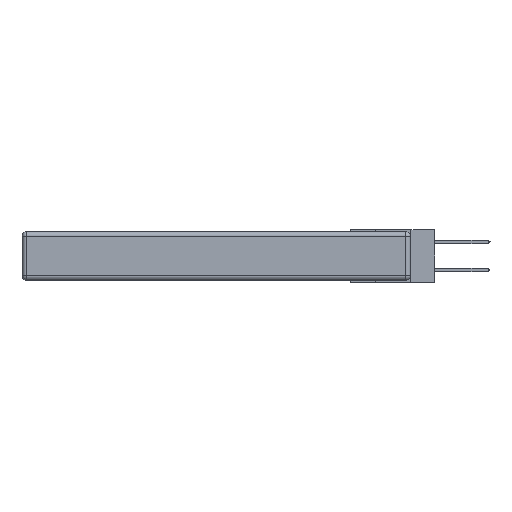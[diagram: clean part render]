
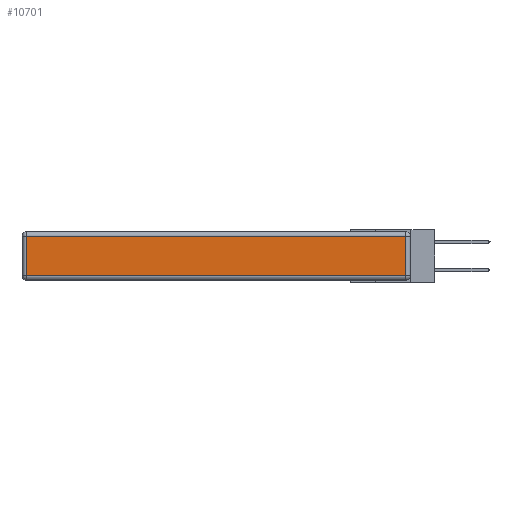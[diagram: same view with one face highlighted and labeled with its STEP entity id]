
A CAD part, left-side view. The second image highlights one B-rep face of the part: STEP entity #10701.
In plain terms, the highlighted planar face has unit normal (-1, 0, 0).
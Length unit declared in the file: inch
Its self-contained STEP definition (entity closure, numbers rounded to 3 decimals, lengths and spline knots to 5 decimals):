
#21 = VECTOR ( 'NONE', #9595, 39.37008 ) ;
#179 = EDGE_CURVE ( 'NONE', #8770, #10755, #1610, .T. ) ;
#392 = VECTOR ( 'NONE', #9634, 39.37008 ) ;
#1179 = EDGE_LOOP ( 'NONE', ( #4653, #8578, #7617, #9391 ) ) ;
#1444 = DIRECTION ( 'NONE',  ( 0., 0., 1. ) ) ;
#1610 = LINE ( 'NONE', #1983, #392 ) ;
#1983 = CARTESIAN_POINT ( 'NONE',  ( 0., 2.72, -0.343 ) ) ;
#4003 = LINE ( 'NONE', #9687, #13252 ) ;
#4013 = CARTESIAN_POINT ( 'NONE',  ( 0., 0.03, -0.313 ) ) ;
#4406 = DIRECTION ( 'NONE',  ( 0., 1., 0. ) ) ;
#4653 = ORIENTED_EDGE ( 'NONE', *, *, #6406, .T. ) ;
#4822 = AXIS2_PLACEMENT_3D ( 'NONE', #11299, #12381, #1444 ) ;
#5662 = PLANE ( 'NONE',  #4822 ) ;
#6313 = LINE ( 'NONE', #11982, #13309 ) ;
#6406 = EDGE_CURVE ( 'NONE', #10755, #13877, #7732, .T. ) ;
#6675 = CARTESIAN_POINT ( 'NONE',  ( 0., 0.03, -0.03 ) ) ;
#7079 = CARTESIAN_POINT ( 'NONE',  ( 0., 2.72, -0.313 ) ) ;
#7617 = ORIENTED_EDGE ( 'NONE', *, *, #10824, .T. ) ;
#7732 = LINE ( 'NONE', #11595, #21 ) ;
#8578 = ORIENTED_EDGE ( 'NONE', *, *, #14036, .T. ) ;
#8770 = VERTEX_POINT ( 'NONE', #10981 ) ;
#9340 = FACE_OUTER_BOUND ( 'NONE', #1179, .T. ) ;
#9391 = ORIENTED_EDGE ( 'NONE', *, *, #179, .T. ) ;
#9595 = DIRECTION ( 'NONE',  ( 0., -1., 0. ) ) ;
#9634 = DIRECTION ( 'NONE',  ( 0., 0., -1. ) ) ;
#9687 = CARTESIAN_POINT ( 'NONE',  ( 0., 2.75, -0.03 ) ) ;
#9796 = DIRECTION ( 'NONE',  ( 0., 0., 1. ) ) ;
#10701 = ADVANCED_FACE ( 'NONE', ( #9340 ), #5662, .T. ) ;
#10755 = VERTEX_POINT ( 'NONE', #7079 ) ;
#10824 = EDGE_CURVE ( 'NONE', #12622, #8770, #4003, .T. ) ;
#10981 = CARTESIAN_POINT ( 'NONE',  ( 0., 2.72, -0.03 ) ) ;
#11299 = CARTESIAN_POINT ( 'NONE',  ( 0., 0., -0.343 ) ) ;
#11595 = CARTESIAN_POINT ( 'NONE',  ( 0., 0., -0.313 ) ) ;
#11982 = CARTESIAN_POINT ( 'NONE',  ( 0., 0.03, -0.343 ) ) ;
#12381 = DIRECTION ( 'NONE',  ( -1., 0., 0. ) ) ;
#12622 = VERTEX_POINT ( 'NONE', #6675 ) ;
#13252 = VECTOR ( 'NONE', #4406, 39.37008 ) ;
#13309 = VECTOR ( 'NONE', #9796, 39.37008 ) ;
#13877 = VERTEX_POINT ( 'NONE', #4013 ) ;
#14036 = EDGE_CURVE ( 'NONE', #13877, #12622, #6313, .T. ) ;
